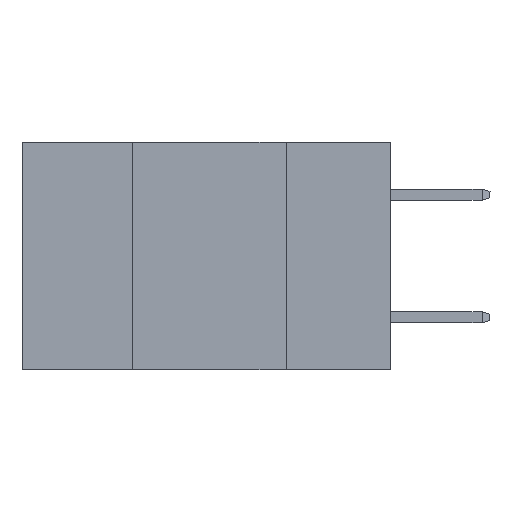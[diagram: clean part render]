
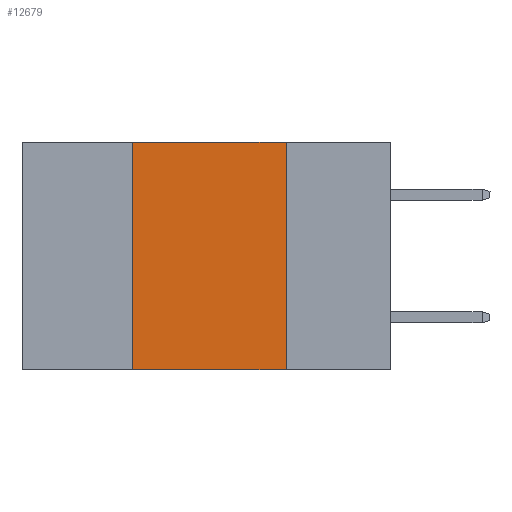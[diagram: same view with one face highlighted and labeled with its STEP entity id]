
A CAD part, left-side view. The second image highlights one B-rep face of the part: STEP entity #12679.
In plain terms, the highlighted planar face has unit normal (-1, 0, 0).
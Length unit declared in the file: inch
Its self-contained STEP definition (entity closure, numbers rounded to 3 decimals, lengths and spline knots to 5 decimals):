
#1324 = EDGE_CURVE ( 'NONE', #6941, #13660, #3228, .T. ) ;
#1484 = DIRECTION ( 'NONE',  ( 0., -1., 0. ) ) ;
#2051 = CARTESIAN_POINT ( 'NONE',  ( 0., 0.17, 0. ) ) ;
#2459 = CARTESIAN_POINT ( 'NONE',  ( 0., 0.17, -0.37 ) ) ;
#2733 = EDGE_CURVE ( 'NONE', #13660, #9579, #9965, .T. ) ;
#3228 = LINE ( 'NONE', #5963, #17066 ) ;
#5963 = CARTESIAN_POINT ( 'NONE',  ( 0., 0.6, 0. ) ) ;
#6036 = EDGE_LOOP ( 'NONE', ( #15340, #13672, #12472, #11795 ) ) ;
#6245 = PLANE ( 'NONE',  #10284 ) ;
#6747 = CARTESIAN_POINT ( 'NONE',  ( 0., 0.42, 0. ) ) ;
#6941 = VERTEX_POINT ( 'NONE', #6747 ) ;
#7308 = DIRECTION ( 'NONE',  ( 0., -1., 0. ) ) ;
#7578 = DIRECTION ( 'NONE',  ( 1., 0., 0. ) ) ;
#8971 = CARTESIAN_POINT ( 'NONE',  ( 0., 0.17, 0. ) ) ;
#9535 = VECTOR ( 'NONE', #10400, 39.37008 ) ;
#9579 = VERTEX_POINT ( 'NONE', #2459 ) ;
#9585 = VECTOR ( 'NONE', #15940, 39.37008 ) ;
#9965 = LINE ( 'NONE', #8971, #9535 ) ;
#10284 = AXIS2_PLACEMENT_3D ( 'NONE', #11594, #7578, #16917 ) ;
#10295 = VERTEX_POINT ( 'NONE', #14915 ) ;
#10400 = DIRECTION ( 'NONE',  ( 0., 0., -1. ) ) ;
#10840 = LINE ( 'NONE', #12378, #14451 ) ;
#11594 = CARTESIAN_POINT ( 'NONE',  ( 0., 0.6, 0. ) ) ;
#11795 = ORIENTED_EDGE ( 'NONE', *, *, #15852, .T. ) ;
#12378 = CARTESIAN_POINT ( 'NONE',  ( 0., 0.6, -0.37 ) ) ;
#12472 = ORIENTED_EDGE ( 'NONE', *, *, #14397, .F. ) ;
#12679 = ADVANCED_FACE ( 'NONE', ( #13202 ), #6245, .F. ) ;
#13202 = FACE_OUTER_BOUND ( 'NONE', #6036, .T. ) ;
#13660 = VERTEX_POINT ( 'NONE', #2051 ) ;
#13672 = ORIENTED_EDGE ( 'NONE', *, *, #1324, .F. ) ;
#14397 = EDGE_CURVE ( 'NONE', #10295, #6941, #16680, .T. ) ;
#14451 = VECTOR ( 'NONE', #1484, 39.37008 ) ;
#14731 = CARTESIAN_POINT ( 'NONE',  ( 0., 0.42, 0. ) ) ;
#14915 = CARTESIAN_POINT ( 'NONE',  ( 0., 0.42, -0.37 ) ) ;
#15340 = ORIENTED_EDGE ( 'NONE', *, *, #2733, .F. ) ;
#15852 = EDGE_CURVE ( 'NONE', #10295, #9579, #10840, .T. ) ;
#15940 = DIRECTION ( 'NONE',  ( 0., 0., 1. ) ) ;
#16680 = LINE ( 'NONE', #14731, #9585 ) ;
#16917 = DIRECTION ( 'NONE',  ( 0., 0., -1. ) ) ;
#17066 = VECTOR ( 'NONE', #7308, 39.37008 ) ;
